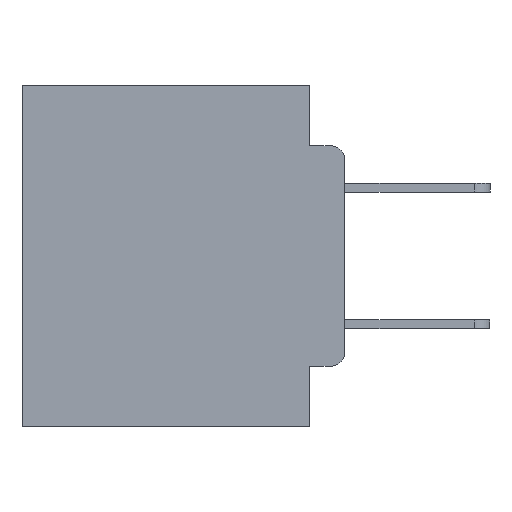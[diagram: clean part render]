
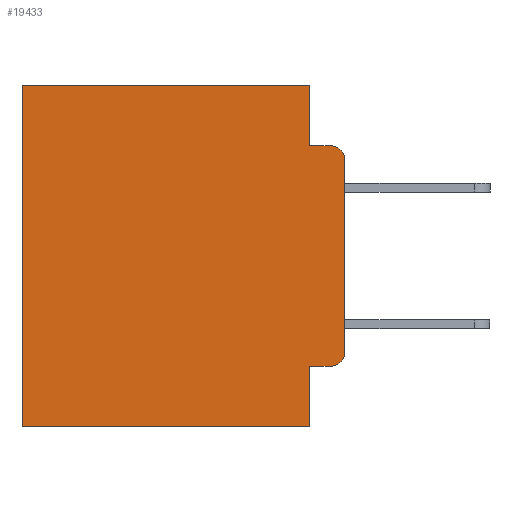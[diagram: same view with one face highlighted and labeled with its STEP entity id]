
A CAD part, left-side view. The second image highlights one B-rep face of the part: STEP entity #19433.
In plain terms, the highlighted planar face has unit normal (-1, 0, 0).
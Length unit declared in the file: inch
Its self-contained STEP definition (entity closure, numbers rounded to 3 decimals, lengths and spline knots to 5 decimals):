
#71 = VERTEX_POINT ( 'NONE', #15897 ) ;
#116 = EDGE_LOOP ( 'NONE', ( #14633, #3348, #14509, #4097, #24129, #8978, #17213, #2684, #20960, #3614 ) ) ;
#1367 = CIRCLE ( 'NONE', #6127, 0.02 ) ;
#1552 = CARTESIAN_POINT ( 'NONE',  ( 0.298, 0., -0.3915 ) ) ;
#2482 = CARTESIAN_POINT ( 'NONE',  ( 0.298, 0., 0. ) ) ;
#2531 = CARTESIAN_POINT ( 'NONE',  ( 0.298, 0.473, 0. ) ) ;
#2640 = CARTESIAN_POINT ( 'NONE',  ( 0.298, 0.051, -0.4115 ) ) ;
#2684 = ORIENTED_EDGE ( 'NONE', *, *, #19683, .F. ) ;
#3348 = ORIENTED_EDGE ( 'NONE', *, *, #17786, .T. ) ;
#3614 = ORIENTED_EDGE ( 'NONE', *, *, #12815, .T. ) ;
#3839 = LINE ( 'NONE', #19026, #25237 ) ;
#4020 = VECTOR ( 'NONE', #21870, 39.37008 ) ;
#4097 = ORIENTED_EDGE ( 'NONE', *, *, #23760, .F. ) ;
#4501 = CARTESIAN_POINT ( 'NONE',  ( 0.298, 0.051, -0.0885 ) ) ;
#4687 = VERTEX_POINT ( 'NONE', #4501 ) ;
#5460 = LINE ( 'NONE', #20088, #15985 ) ;
#5477 = VERTEX_POINT ( 'NONE', #19995 ) ;
#5532 = DIRECTION ( 'NONE',  ( 0., 0., -1. ) ) ;
#5558 = CARTESIAN_POINT ( 'NONE',  ( 0.298, 0.02, -0.1085 ) ) ;
#5843 = VECTOR ( 'NONE', #15315, 39.37008 ) ;
#6127 = AXIS2_PLACEMENT_3D ( 'NONE', #5558, #20117, #7735 ) ;
#6234 = CARTESIAN_POINT ( 'NONE',  ( 0.298, 0.051, 0. ) ) ;
#6521 = LINE ( 'NONE', #23187, #12773 ) ;
#7530 = VERTEX_POINT ( 'NONE', #26667 ) ;
#7735 = DIRECTION ( 'NONE',  ( 0., 0., -1. ) ) ;
#7884 = CARTESIAN_POINT ( 'NONE',  ( 0.298, 0.051, -0.0885 ) ) ;
#7994 = CARTESIAN_POINT ( 'NONE',  ( 0.298, 0.051, -0.4115 ) ) ;
#8791 = EDGE_CURVE ( 'NONE', #23115, #25430, #3839, .T. ) ;
#8978 = ORIENTED_EDGE ( 'NONE', *, *, #21063, .T. ) ;
#9545 = CARTESIAN_POINT ( 'NONE',  ( 0.298, 0.473, 0. ) ) ;
#9948 = VERTEX_POINT ( 'NONE', #13675 ) ;
#11052 = PLANE ( 'NONE',  #21626 ) ;
#11295 = CARTESIAN_POINT ( 'NONE',  ( 0.298, 0.02, -0.3915 ) ) ;
#12401 = FACE_OUTER_BOUND ( 'NONE', #116, .T. ) ;
#12509 = DIRECTION ( 'NONE',  ( 0., 0., -1. ) ) ;
#12527 = VERTEX_POINT ( 'NONE', #1552 ) ;
#12773 = VECTOR ( 'NONE', #17042, 39.37008 ) ;
#12815 = EDGE_CURVE ( 'NONE', #5477, #12527, #20855, .T. ) ;
#13198 = DIRECTION ( 'NONE',  ( 0., 0., -1. ) ) ;
#13342 = DIRECTION ( 'NONE',  ( 0., 0., -1. ) ) ;
#13675 = CARTESIAN_POINT ( 'NONE',  ( 0.298, 0.473, -0.5 ) ) ;
#13859 = LINE ( 'NONE', #6234, #18029 ) ;
#14509 = ORIENTED_EDGE ( 'NONE', *, *, #25084, .F. ) ;
#14541 = EDGE_CURVE ( 'NONE', #7530, #12527, #6521, .T. ) ;
#14633 = ORIENTED_EDGE ( 'NONE', *, *, #14541, .F. ) ;
#15315 = DIRECTION ( 'NONE',  ( 0., -1., 0. ) ) ;
#15897 = CARTESIAN_POINT ( 'NONE',  ( 0.298, 0.051, -0.5 ) ) ;
#15985 = VECTOR ( 'NONE', #5532, 39.37008 ) ;
#17042 = DIRECTION ( 'NONE',  ( 0., 0., -1. ) ) ;
#17213 = ORIENTED_EDGE ( 'NONE', *, *, #26260, .F. ) ;
#17786 = EDGE_CURVE ( 'NONE', #7530, #23541, #1367, .T. ) ;
#18029 = VECTOR ( 'NONE', #12509, 39.37008 ) ;
#18184 = DIRECTION ( 'NONE',  ( 0., -1., 0. ) ) ;
#18237 = VECTOR ( 'NONE', #25989, 39.37008 ) ;
#18269 = CARTESIAN_POINT ( 'NONE',  ( 0.298, 0.051, 0. ) ) ;
#18305 = EDGE_CURVE ( 'NONE', #24588, #5477, #27051, .T. ) ;
#19026 = CARTESIAN_POINT ( 'NONE',  ( 0.298, 0., 0. ) ) ;
#19433 = ADVANCED_FACE ( 'NONE', ( #12401 ), #11052, .F. ) ;
#19683 = EDGE_CURVE ( 'NONE', #24588, #71, #5460, .T. ) ;
#19755 = DIRECTION ( 'NONE',  ( 0., 1., 0. ) ) ;
#19995 = CARTESIAN_POINT ( 'NONE',  ( 0.298, 0.02, -0.4115 ) ) ;
#20088 = CARTESIAN_POINT ( 'NONE',  ( 0.298, 0.051, 0. ) ) ;
#20117 = DIRECTION ( 'NONE',  ( -1., 0., 0. ) ) ;
#20690 = LINE ( 'NONE', #9545, #4020 ) ;
#20855 = CIRCLE ( 'NONE', #22393, 0.02 ) ;
#20960 = ORIENTED_EDGE ( 'NONE', *, *, #18305, .T. ) ;
#21063 = EDGE_CURVE ( 'NONE', #25430, #9948, #20690, .T. ) ;
#21626 = AXIS2_PLACEMENT_3D ( 'NONE', #2482, #25369, #13198 ) ;
#21870 = DIRECTION ( 'NONE',  ( 0., 0., -1. ) ) ;
#22004 = CARTESIAN_POINT ( 'NONE',  ( 0.298, 0.02, -0.0885 ) ) ;
#22109 = LINE ( 'NONE', #7884, #26781 ) ;
#22393 = AXIS2_PLACEMENT_3D ( 'NONE', #11295, #25524, #13342 ) ;
#23115 = VERTEX_POINT ( 'NONE', #18269 ) ;
#23187 = CARTESIAN_POINT ( 'NONE',  ( 0.298, 0., 0. ) ) ;
#23541 = VERTEX_POINT ( 'NONE', #22004 ) ;
#23760 = EDGE_CURVE ( 'NONE', #23115, #4687, #13859, .T. ) ;
#23997 = CARTESIAN_POINT ( 'NONE',  ( 0.298, 0., -0.5 ) ) ;
#24129 = ORIENTED_EDGE ( 'NONE', *, *, #8791, .T. ) ;
#24275 = LINE ( 'NONE', #23997, #18237 ) ;
#24588 = VERTEX_POINT ( 'NONE', #7994 ) ;
#25084 = EDGE_CURVE ( 'NONE', #4687, #23541, #22109, .T. ) ;
#25237 = VECTOR ( 'NONE', #19755, 39.37008 ) ;
#25369 = DIRECTION ( 'NONE',  ( 1., 0., 0. ) ) ;
#25430 = VERTEX_POINT ( 'NONE', #2531 ) ;
#25524 = DIRECTION ( 'NONE',  ( -1., 0., 0. ) ) ;
#25989 = DIRECTION ( 'NONE',  ( 0., 1., 0. ) ) ;
#26260 = EDGE_CURVE ( 'NONE', #71, #9948, #24275, .T. ) ;
#26667 = CARTESIAN_POINT ( 'NONE',  ( 0.298, 0., -0.1085 ) ) ;
#26781 = VECTOR ( 'NONE', #18184, 39.37008 ) ;
#27051 = LINE ( 'NONE', #2640, #5843 ) ;
